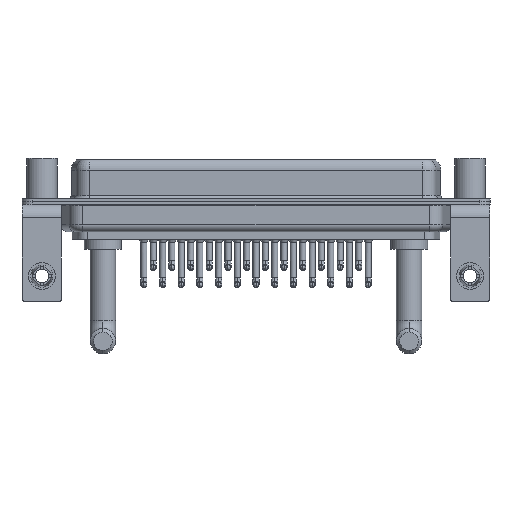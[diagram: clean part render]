
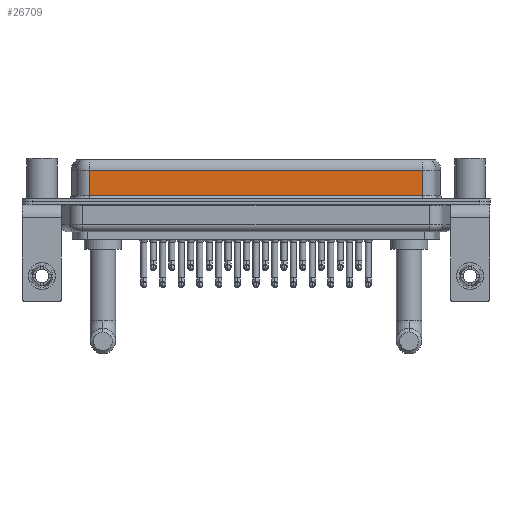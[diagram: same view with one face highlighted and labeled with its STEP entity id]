
A CAD part, front view. The second image highlights one B-rep face of the part: STEP entity #26709.
In plain terms, the highlighted planar face has unit normal (0, -1, 0).
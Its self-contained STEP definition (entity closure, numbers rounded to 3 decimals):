
#1299 = VERTEX_POINT ( 'NONE', #12550 ) ;
#2397 = AXIS2_PLACEMENT_3D ( 'NONE', #18066, #13253, #22188 ) ;
#2637 = CARTESIAN_POINT ( 'NONE',  ( 56.462, -3.95, 4.65 ) ) ;
#3112 = VERTEX_POINT ( 'NONE', #5361 ) ;
#4164 = FACE_OUTER_BOUND ( 'NONE', #23261, .T. ) ;
#4879 = LINE ( 'NONE', #5147, #26278 ) ;
#4978 = CARTESIAN_POINT ( 'NONE',  ( 56.462, -3.95, 0.9 ) ) ;
#5147 = CARTESIAN_POINT ( 'NONE',  ( 56.462, -3.95, 6.4 ) ) ;
#5361 = CARTESIAN_POINT ( 'NONE',  ( 56.462, -3.95, 0.9 ) ) ;
#5544 = VERTEX_POINT ( 'NONE', #2637 ) ;
#5545 = LINE ( 'NONE', #4978, #7347 ) ;
#6025 = CARTESIAN_POINT ( 'NONE',  ( 7.038, -3.95, 6.4 ) ) ;
#6930 = EDGE_CURVE ( 'NONE', #1299, #3112, #5545, .T. ) ;
#7347 = VECTOR ( 'NONE', #13909, 1000. ) ;
#8380 = VECTOR ( 'NONE', #19643, 1000. ) ;
#8717 = PLANE ( 'NONE',  #2397 ) ;
#9504 = ORIENTED_EDGE ( 'NONE', *, *, #6930, .T. ) ;
#10875 = EDGE_CURVE ( 'NONE', #5544, #3112, #4879, .T. ) ;
#11263 = CARTESIAN_POINT ( 'NONE',  ( 7.038, -3.95, 4.65 ) ) ;
#12550 = CARTESIAN_POINT ( 'NONE',  ( 7.038, -3.95, 0.9 ) ) ;
#13253 = DIRECTION ( 'NONE',  ( 0., 1., 0. ) ) ;
#13700 = ORIENTED_EDGE ( 'NONE', *, *, #17711, .T. ) ;
#13807 = DIRECTION ( 'NONE',  ( 0., 0., -1. ) ) ;
#13909 = DIRECTION ( 'NONE',  ( 1., 0., 0. ) ) ;
#15778 = ORIENTED_EDGE ( 'NONE', *, *, #10875, .F. ) ;
#17711 = EDGE_CURVE ( 'NONE', #24431, #1299, #26236, .T. ) ;
#18066 = CARTESIAN_POINT ( 'NONE',  ( 56.462, -3.95, 6.4 ) ) ;
#18932 = ORIENTED_EDGE ( 'NONE', *, *, #19665, .T. ) ;
#19056 = LINE ( 'NONE', #26106, #8380 ) ;
#19643 = DIRECTION ( 'NONE',  ( -1., 0., 0. ) ) ;
#19665 = EDGE_CURVE ( 'NONE', #5544, #24431, #19056, .T. ) ;
#22188 = DIRECTION ( 'NONE',  ( 0., 0., 1. ) ) ;
#23261 = EDGE_LOOP ( 'NONE', ( #15778, #18932, #13700, #9504 ) ) ;
#24168 = DIRECTION ( 'NONE',  ( 0., 0., -1. ) ) ;
#24431 = VERTEX_POINT ( 'NONE', #11263 ) ;
#26106 = CARTESIAN_POINT ( 'NONE',  ( 56.462, -3.95, 4.65 ) ) ;
#26236 = LINE ( 'NONE', #6025, #26670 ) ;
#26278 = VECTOR ( 'NONE', #13807, 1000. ) ;
#26670 = VECTOR ( 'NONE', #24168, 1000. ) ;
#26709 = ADVANCED_FACE ( 'NONE', ( #4164 ), #8717, .F. ) ;
